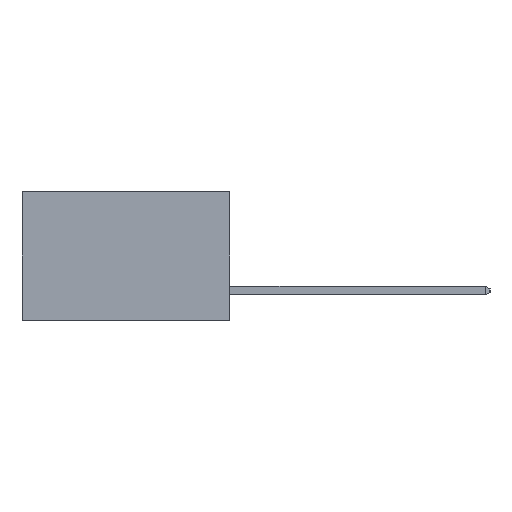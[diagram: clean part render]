
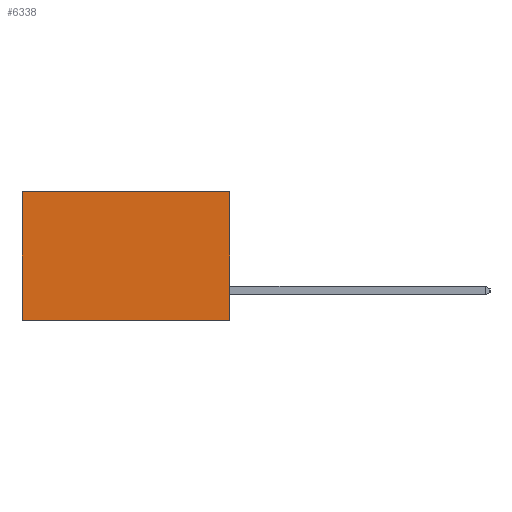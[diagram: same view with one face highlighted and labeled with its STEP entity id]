
A CAD part, left-side view. The second image highlights one B-rep face of the part: STEP entity #6338.
In plain terms, the highlighted planar face has unit normal (-1, 0, 0).
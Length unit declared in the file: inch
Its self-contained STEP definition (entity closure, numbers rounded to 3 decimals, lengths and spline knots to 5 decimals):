
#3605 = ORIENTED_EDGE ( 'NONE', *, *, #11862, .F. ) ;
#3762 = ORIENTED_EDGE ( 'NONE', *, *, #25520, .F. ) ;
#4707 = CARTESIAN_POINT ( 'NONE',  ( 0.298, 0.6, -0.37 ) ) ;
#4930 = LINE ( 'NONE', #10743, #25443 ) ;
#5835 = VERTEX_POINT ( 'NONE', #8885 ) ;
#6338 = ADVANCED_FACE ( 'NONE', ( #14606 ), #23474, .F. ) ;
#6614 = DIRECTION ( 'NONE',  ( 0., 0., -1. ) ) ;
#6794 = DIRECTION ( 'NONE',  ( 0., 1., 0. ) ) ;
#7339 = EDGE_CURVE ( 'NONE', #19309, #24120, #10190, .T. ) ;
#7699 = CARTESIAN_POINT ( 'NONE',  ( 0.298, 0.6, 0. ) ) ;
#8885 = CARTESIAN_POINT ( 'NONE',  ( 0.298, 0., -0.37 ) ) ;
#9293 = ORIENTED_EDGE ( 'NONE', *, *, #7339, .T. ) ;
#9352 = CARTESIAN_POINT ( 'NONE',  ( 0.298, 0., 0. ) ) ;
#10190 = LINE ( 'NONE', #16851, #25303 ) ;
#10743 = CARTESIAN_POINT ( 'NONE',  ( 0.298, 0., -0.37 ) ) ;
#11378 = DIRECTION ( 'NONE',  ( 0., 1., 0. ) ) ;
#11862 = EDGE_CURVE ( 'NONE', #5835, #24120, #4930, .T. ) ;
#11916 = VECTOR ( 'NONE', #11378, 39.37008 ) ;
#13531 = ORIENTED_EDGE ( 'NONE', *, *, #18496, .T. ) ;
#14598 = VERTEX_POINT ( 'NONE', #15964 ) ;
#14606 = FACE_OUTER_BOUND ( 'NONE', #25613, .T. ) ;
#14745 = CARTESIAN_POINT ( 'NONE',  ( 0.298, 0., 0. ) ) ;
#14946 = AXIS2_PLACEMENT_3D ( 'NONE', #23496, #17100, #17075 ) ;
#15964 = CARTESIAN_POINT ( 'NONE',  ( 0.298, 0., 0. ) ) ;
#16257 = LINE ( 'NONE', #14745, #25401 ) ;
#16851 = CARTESIAN_POINT ( 'NONE',  ( 0.298, 0.6, 0. ) ) ;
#17075 = DIRECTION ( 'NONE',  ( 0., 0., -1. ) ) ;
#17100 = DIRECTION ( 'NONE',  ( 1., 0., 0. ) ) ;
#17235 = LINE ( 'NONE', #9352, #11916 ) ;
#18496 = EDGE_CURVE ( 'NONE', #14598, #19309, #17235, .T. ) ;
#19309 = VERTEX_POINT ( 'NONE', #7699 ) ;
#20734 = DIRECTION ( 'NONE',  ( 0., 0., -1. ) ) ;
#23474 = PLANE ( 'NONE',  #14946 ) ;
#23496 = CARTESIAN_POINT ( 'NONE',  ( 0.298, 0., 0. ) ) ;
#24120 = VERTEX_POINT ( 'NONE', #4707 ) ;
#25303 = VECTOR ( 'NONE', #6614, 39.37008 ) ;
#25401 = VECTOR ( 'NONE', #20734, 39.37008 ) ;
#25443 = VECTOR ( 'NONE', #6794, 39.37008 ) ;
#25520 = EDGE_CURVE ( 'NONE', #14598, #5835, #16257, .T. ) ;
#25613 = EDGE_LOOP ( 'NONE', ( #9293, #3605, #3762, #13531 ) ) ;
